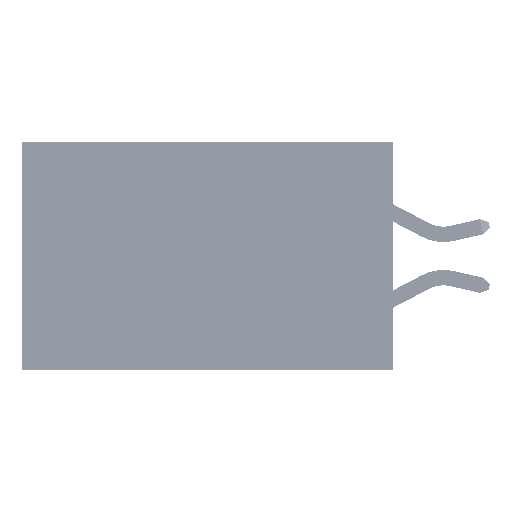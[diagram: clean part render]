
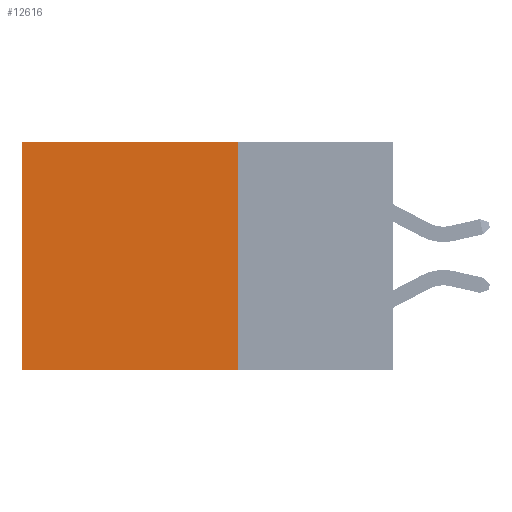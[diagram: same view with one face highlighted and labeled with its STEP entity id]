
A CAD part, left-side view. The second image highlights one B-rep face of the part: STEP entity #12616.
In plain terms, the highlighted planar face has unit normal (-1, 0, 0).
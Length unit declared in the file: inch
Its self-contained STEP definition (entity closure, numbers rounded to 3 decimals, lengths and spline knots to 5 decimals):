
#4 = CARTESIAN_POINT ( 'NONE',  ( 0.2875, 0.25, 0. ) ) ;
#123 = DIRECTION ( 'NONE',  ( 1., 0., 0. ) ) ;
#282 = EDGE_CURVE ( 'NONE', #33763, #21333, #7262, .T. ) ;
#806 = CARTESIAN_POINT ( 'NONE',  ( 0.2875, 0.6, 0. ) ) ;
#4161 = EDGE_CURVE ( 'NONE', #21333, #40321, #12459, .T. ) ;
#7262 = LINE ( 'NONE', #14580, #32601 ) ;
#7667 = DIRECTION ( 'NONE',  ( 0., 1., 0. ) ) ;
#8517 = DIRECTION ( 'NONE',  ( 0., 0., -1. ) ) ;
#9075 = PLANE ( 'NONE',  #30479 ) ;
#11077 = LINE ( 'NONE', #39063, #32190 ) ;
#12459 = LINE ( 'NONE', #23965, #14052 ) ;
#12466 = CARTESIAN_POINT ( 'NONE',  ( 0.2875, 0.25, 0. ) ) ;
#12616 = ADVANCED_FACE ( 'NONE', ( #28213 ), #9075, .F. ) ;
#13989 = ORIENTED_EDGE ( 'NONE', *, *, #25609, .T. ) ;
#14052 = VECTOR ( 'NONE', #33883, 39.37008 ) ;
#14580 = CARTESIAN_POINT ( 'NONE',  ( 0.2875, 0.25, 0. ) ) ;
#16611 = EDGE_CURVE ( 'NONE', #33763, #35200, #22817, .T. ) ;
#16706 = CARTESIAN_POINT ( 'NONE',  ( 0.2875, 0.25, -0.37 ) ) ;
#16811 = DIRECTION ( 'NONE',  ( 0., 0., -1. ) ) ;
#17667 = ORIENTED_EDGE ( 'NONE', *, *, #282, .F. ) ;
#18247 = CARTESIAN_POINT ( 'NONE',  ( 0.2875, 0.25, 0. ) ) ;
#21290 = ORIENTED_EDGE ( 'NONE', *, *, #4161, .F. ) ;
#21333 = VERTEX_POINT ( 'NONE', #16706 ) ;
#22817 = LINE ( 'NONE', #18247, #24920 ) ;
#23940 = CARTESIAN_POINT ( 'NONE',  ( 0.2875, 0.6, -0.37 ) ) ;
#23965 = CARTESIAN_POINT ( 'NONE',  ( 0.2875, 0.25, -0.37 ) ) ;
#24920 = VECTOR ( 'NONE', #7667, 39.37008 ) ;
#25609 = EDGE_CURVE ( 'NONE', #35200, #40321, #11077, .T. ) ;
#28213 = FACE_OUTER_BOUND ( 'NONE', #43109, .T. ) ;
#30479 = AXIS2_PLACEMENT_3D ( 'NONE', #12466, #123, #16811 ) ;
#31704 = DIRECTION ( 'NONE',  ( 0., 0., -1. ) ) ;
#32190 = VECTOR ( 'NONE', #8517, 39.37008 ) ;
#32601 = VECTOR ( 'NONE', #31704, 39.37008 ) ;
#33763 = VERTEX_POINT ( 'NONE', #4 ) ;
#33883 = DIRECTION ( 'NONE',  ( 0., 1., 0. ) ) ;
#35200 = VERTEX_POINT ( 'NONE', #806 ) ;
#37835 = ORIENTED_EDGE ( 'NONE', *, *, #16611, .T. ) ;
#39063 = CARTESIAN_POINT ( 'NONE',  ( 0.2875, 0.6, 0. ) ) ;
#40321 = VERTEX_POINT ( 'NONE', #23940 ) ;
#43109 = EDGE_LOOP ( 'NONE', ( #13989, #21290, #17667, #37835 ) ) ;
